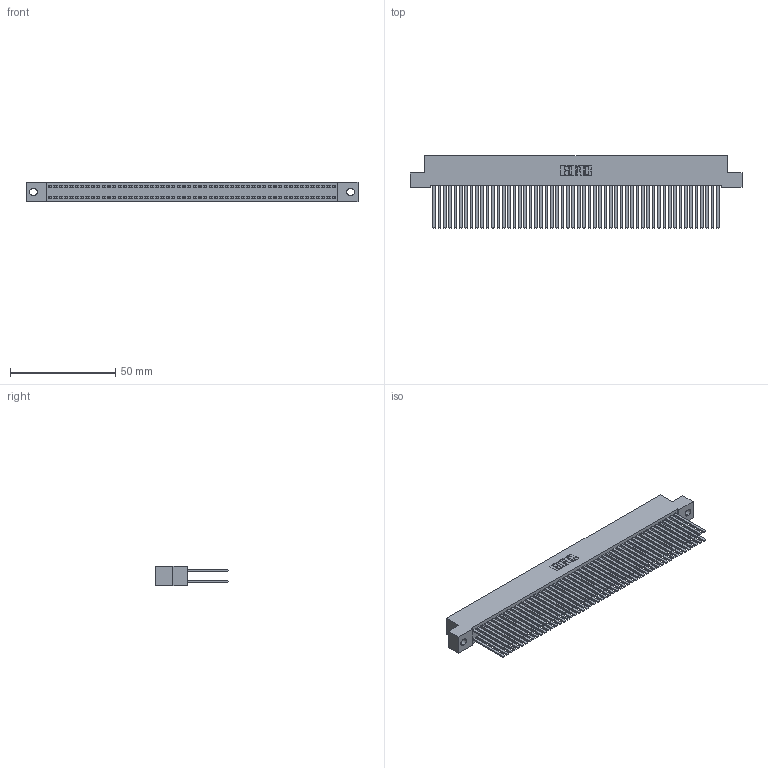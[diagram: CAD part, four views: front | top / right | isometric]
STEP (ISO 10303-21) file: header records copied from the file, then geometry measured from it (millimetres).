
FILE_DESCRIPTION (( 'STEP AP203' ), '1' );
FILE_NAME ('342-108-544-202.STEP', '2019-10-04T19:52:05', ( '' ), ( '' ), 'SwSTEP 2.0', 'SolidWorks 2016', '' );
FILE_SCHEMA (( 'CONFIG_CONTROL_DESIGN' ));
Length unit declared in the file: inch
Products named in the file (3): 345-292-001_345-293-144; 342-108-544-202; 342 Part_.128 Slot
Assembly tree (109 placements, depth 2):
  342-108-544-202
    342 Part_.128 Slot
    345-292-001_345-293-144  x108
Bounding box: 157.48 x 34.3 x 9.4 mm (x, y, z)
Volume: 15668.2 mm3; surface area: 29751.7 mm2
Topology: 109 solids, 109 shells, 5082 faces, 15107 edges, 9926 vertices
Faces by surface type: plane 3526, cylinder 1556
Entity records: 33007 total; most frequent: CARTESIAN_POINT 5454, ORIENTED_EDGE 5390, DIRECTION 4635, EDGE_CURVE 2695, VECTOR 2571, LINE 2571, VERTEX_POINT 1794, AXIS2_PLACEMENT_3D 1032
